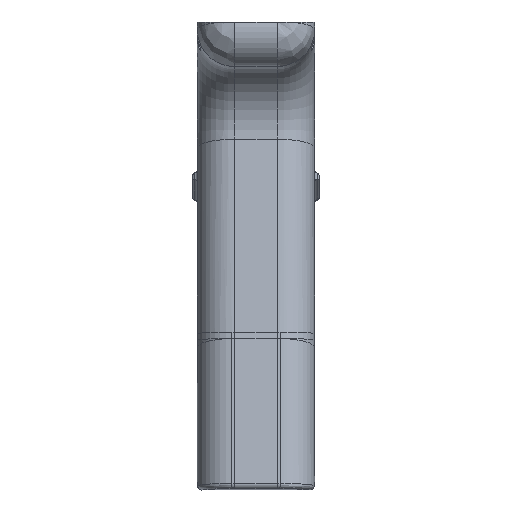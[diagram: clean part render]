
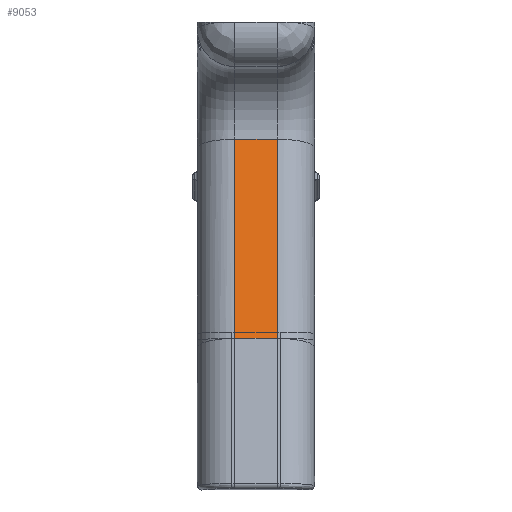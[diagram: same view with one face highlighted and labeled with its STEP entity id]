
A CAD part, front view. The second image highlights one B-rep face of the part: STEP entity #9053.
In plain terms, the highlighted face is planar.
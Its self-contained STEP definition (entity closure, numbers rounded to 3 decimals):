
#857=PLANE('',#9875);
#1263=FACE_OUTER_BOUND('',#1783,.T.);
#1783=EDGE_LOOP('',(#7803,#7804,#7805,#7806));
#2387=LINE('',#16018,#3130);
#2545=LINE('',#16872,#3288);
#2546=LINE('',#16875,#3289);
#2547=LINE('',#16876,#3290);
#3130=VECTOR('',#11543,10.);
#3288=VECTOR('',#11949,10.);
#3289=VECTOR('',#11952,10.);
#3290=VECTOR('',#11953,10.);
#4185=VERTEX_POINT('',#16014);
#4186=VERTEX_POINT('',#16016);
#4325=VERTEX_POINT('',#16850);
#4328=VERTEX_POINT('',#16874);
#5324=EDGE_CURVE('',#4185,#4186,#2387,.T.);
#5552=EDGE_CURVE('',#4185,#4325,#2545,.T.);
#5553=EDGE_CURVE('',#4328,#4186,#2546,.T.);
#5554=EDGE_CURVE('',#4325,#4328,#2547,.T.);
#7803=ORIENTED_EDGE('',*,*,#5553,.F.);
#7804=ORIENTED_EDGE('',*,*,#5554,.F.);
#7805=ORIENTED_EDGE('',*,*,#5552,.F.);
#7806=ORIENTED_EDGE('',*,*,#5324,.T.);
#9053=ADVANCED_FACE('',(#1263),#857,.T.);
#9875=AXIS2_PLACEMENT_3D('',#16873,#11950,#11951);
#11543=DIRECTION('',(0.,-0.249,0.969));
#11949=DIRECTION('',(-1.,0.,0.));
#11950=DIRECTION('center_axis',(0.,-0.969,
-0.249));
#11951=DIRECTION('ref_axis',(0.,-0.249,0.969));
#11952=DIRECTION('',(1.,0.,0.));
#11953=DIRECTION('',(0.,-0.249,0.969));
#16014=CARTESIAN_POINT('',(13.45,-71.634,19.877));
#16016=CARTESIAN_POINT('',(13.45,-83.628,66.536));
#16018=CARTESIAN_POINT('',(13.45,-83.554,66.245));
#16850=CARTESIAN_POINT('',(3.45,-71.634,19.877));
#16872=CARTESIAN_POINT('',(22.175,-71.634,19.877));
#16873=CARTESIAN_POINT('Origin',(22.175,-71.634,19.877));
#16874=CARTESIAN_POINT('',(3.45,-83.628,66.536));
#16875=CARTESIAN_POINT('',(22.175,-83.628,66.536));
#16876=CARTESIAN_POINT('',(3.45,-83.554,66.245));
